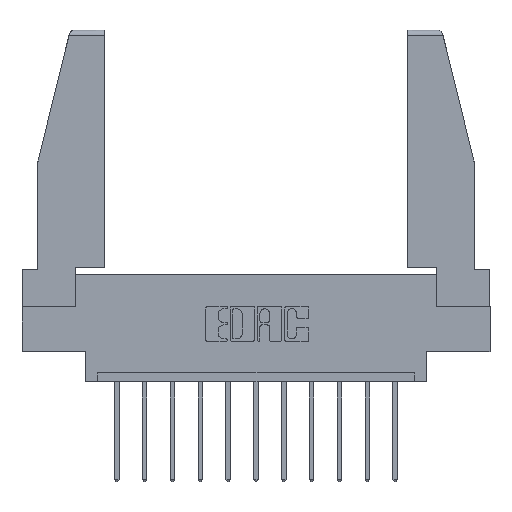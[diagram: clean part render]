
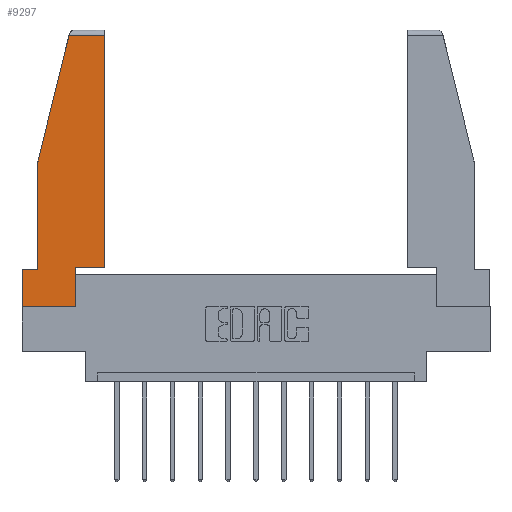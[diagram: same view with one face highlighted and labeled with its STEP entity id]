
A CAD part, top view. The second image highlights one B-rep face of the part: STEP entity #9297.
In plain terms, the highlighted planar face has unit normal (0, 0, 1).
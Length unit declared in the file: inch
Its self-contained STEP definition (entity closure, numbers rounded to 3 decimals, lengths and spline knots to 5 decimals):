
#368 = VERTEX_POINT ( 'NONE', #1755 ) ;
#410 = ORIENTED_EDGE ( 'NONE', *, *, #12310, .T. ) ;
#507 = CARTESIAN_POINT ( 'NONE',  ( 0., 0., 0. ) ) ;
#640 = LINE ( 'NONE', #13456, #6681 ) ;
#1020 = VECTOR ( 'NONE', #5619, 39.37008 ) ;
#1755 = CARTESIAN_POINT ( 'NONE',  ( 0.086, 0.21, 0. ) ) ;
#1830 = CARTESIAN_POINT ( 'NONE',  ( 0.461, 0.223, 0. ) ) ;
#1871 = DIRECTION ( 'NONE',  ( 0., 1., 0. ) ) ;
#2064 = ORIENTED_EDGE ( 'NONE', *, *, #10599, .T. ) ;
#2118 = VECTOR ( 'NONE', #5674, 39.37008 ) ;
#2382 = CARTESIAN_POINT ( 'NONE',  ( 0., 0.21, 0. ) ) ;
#2437 = EDGE_CURVE ( 'NONE', #3087, #10244, #9486, .T. ) ;
#2535 = CARTESIAN_POINT ( 'NONE',  ( 0.461, 1.52, 0. ) ) ;
#2592 = CARTESIAN_POINT ( 'NONE',  ( 0.271, 1.55, 0. ) ) ;
#2642 = LINE ( 'NONE', #2592, #10126 ) ;
#2932 = DIRECTION ( 'NONE',  ( 1., 0., 0. ) ) ;
#2945 = VECTOR ( 'NONE', #1871, 39.37008 ) ;
#3087 = VERTEX_POINT ( 'NONE', #14511 ) ;
#3113 = CARTESIAN_POINT ( 'NONE',  ( 0.297, 0.223, 0. ) ) ;
#3237 = VECTOR ( 'NONE', #11898, 39.37008 ) ;
#3948 = LINE ( 'NONE', #7458, #11989 ) ;
#3954 = ORIENTED_EDGE ( 'NONE', *, *, #7551, .T. ) ;
#3981 = VERTEX_POINT ( 'NONE', #9557 ) ;
#4259 = DIRECTION ( 'NONE',  ( -1., 0., 0. ) ) ;
#4270 = ORIENTED_EDGE ( 'NONE', *, *, #6470, .T. ) ;
#4292 = EDGE_CURVE ( 'NONE', #10625, #3981, #2642, .T. ) ;
#5056 = DIRECTION ( 'NONE',  ( 0., 0., 1. ) ) ;
#5178 = LINE ( 'NONE', #9151, #2118 ) ;
#5593 = VERTEX_POINT ( 'NONE', #10395 ) ;
#5619 = DIRECTION ( 'NONE',  ( 0., 1., 0. ) ) ;
#5674 = DIRECTION ( 'NONE',  ( 0., -1., 0. ) ) ;
#6189 = EDGE_CURVE ( 'NONE', #3981, #368, #12056, .T. ) ;
#6357 = FACE_OUTER_BOUND ( 'NONE', #8509, .T. ) ;
#6470 = EDGE_CURVE ( 'NONE', #10564, #5593, #3948, .T. ) ;
#6611 = VERTEX_POINT ( 'NONE', #10735 ) ;
#6681 = VECTOR ( 'NONE', #4259, 39.37008 ) ;
#6807 = ORIENTED_EDGE ( 'NONE', *, *, #4292, .T. ) ;
#6955 = AXIS2_PLACEMENT_3D ( 'NONE', #13108, #5056, #14200 ) ;
#7307 = CARTESIAN_POINT ( 'NONE',  ( 0.086, 0.8, 0. ) ) ;
#7388 = EDGE_CURVE ( 'NONE', #6611, #3087, #5178, .T. ) ;
#7458 = CARTESIAN_POINT ( 'NONE',  ( 0.297, 0.223, 0. ) ) ;
#7551 = EDGE_CURVE ( 'NONE', #10244, #10564, #10139, .T. ) ;
#7776 = VERTEX_POINT ( 'NONE', #2535 ) ;
#8509 = EDGE_LOOP ( 'NONE', ( #2064, #9277, #6807, #10776, #410, #9930, #8906, #3954, #4270 ) ) ;
#8751 = EDGE_CURVE ( 'NONE', #7776, #10625, #640, .T. ) ;
#8906 = ORIENTED_EDGE ( 'NONE', *, *, #2437, .T. ) ;
#9151 = CARTESIAN_POINT ( 'NONE',  ( 0., 0.21, 0. ) ) ;
#9277 = ORIENTED_EDGE ( 'NONE', *, *, #8751, .T. ) ;
#9297 = ADVANCED_FACE ( 'NONE', ( #6357 ), #14155, .T. ) ;
#9486 = LINE ( 'NONE', #507, #3237 ) ;
#9557 = CARTESIAN_POINT ( 'NONE',  ( 0.086, 0.8, 0. ) ) ;
#9743 = DIRECTION ( 'NONE',  ( 0., -1., 0. ) ) ;
#9930 = ORIENTED_EDGE ( 'NONE', *, *, #7388, .T. ) ;
#10074 = LINE ( 'NONE', #1830, #2945 ) ;
#10126 = VECTOR ( 'NONE', #11737, 39.37008 ) ;
#10139 = LINE ( 'NONE', #10215, #1020 ) ;
#10215 = CARTESIAN_POINT ( 'NONE',  ( 0.297, 0., 0. ) ) ;
#10244 = VERTEX_POINT ( 'NONE', #12927 ) ;
#10387 = VECTOR ( 'NONE', #12789, 39.37008 ) ;
#10395 = CARTESIAN_POINT ( 'NONE',  ( 0.461, 0.223, 0. ) ) ;
#10564 = VERTEX_POINT ( 'NONE', #3113 ) ;
#10599 = EDGE_CURVE ( 'NONE', #5593, #7776, #10074, .T. ) ;
#10625 = VERTEX_POINT ( 'NONE', #11374 ) ;
#10735 = CARTESIAN_POINT ( 'NONE',  ( 0., 0.21, 0. ) ) ;
#10776 = ORIENTED_EDGE ( 'NONE', *, *, #6189, .T. ) ;
#11374 = CARTESIAN_POINT ( 'NONE',  ( 0.2636, 1.52, 0. ) ) ;
#11737 = DIRECTION ( 'NONE',  ( -0.239, -0.971, 0. ) ) ;
#11831 = LINE ( 'NONE', #2382, #10387 ) ;
#11898 = DIRECTION ( 'NONE',  ( 1., 0., 0. ) ) ;
#11989 = VECTOR ( 'NONE', #2932, 39.37008 ) ;
#12056 = LINE ( 'NONE', #7307, #12774 ) ;
#12310 = EDGE_CURVE ( 'NONE', #368, #6611, #11831, .T. ) ;
#12774 = VECTOR ( 'NONE', #9743, 39.37008 ) ;
#12789 = DIRECTION ( 'NONE',  ( -1., 0., 0. ) ) ;
#12927 = CARTESIAN_POINT ( 'NONE',  ( 0.297, 0., 0. ) ) ;
#13108 = CARTESIAN_POINT ( 'NONE',  ( 0., 0., 0. ) ) ;
#13456 = CARTESIAN_POINT ( 'NONE',  ( 0., 1.52, 0. ) ) ;
#14155 = PLANE ( 'NONE',  #6955 ) ;
#14200 = DIRECTION ( 'NONE',  ( 1., 0., 0. ) ) ;
#14511 = CARTESIAN_POINT ( 'NONE',  ( 0., 0., 0. ) ) ;
